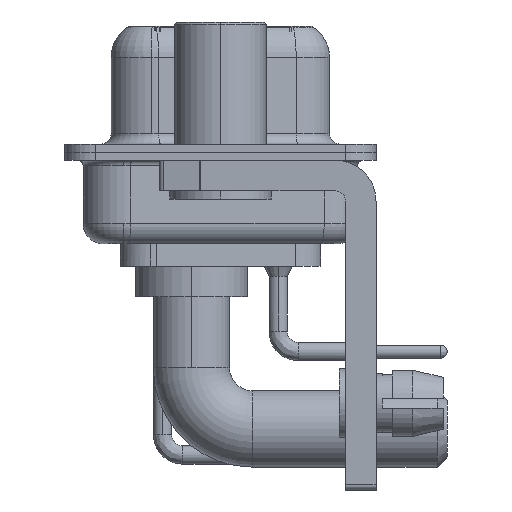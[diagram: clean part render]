
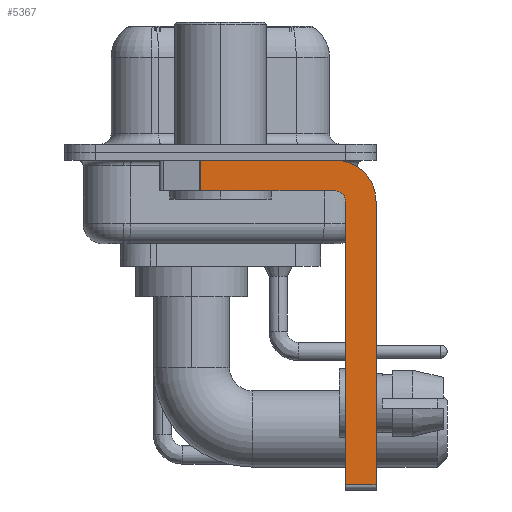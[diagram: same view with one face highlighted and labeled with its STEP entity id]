
A CAD part, left-side view. The second image highlights one B-rep face of the part: STEP entity #5367.
In plain terms, the highlighted planar face has unit normal (-1, 0, 0).
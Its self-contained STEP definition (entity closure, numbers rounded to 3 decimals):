
#263 = ORIENTED_EDGE ( 'NONE', *, *, #15345, .F. ) ;
#335 = EDGE_CURVE ( 'NONE', #21127, #31980, #16540, .T. ) ;
#411 = CARTESIAN_POINT ( 'NONE',  ( -2.9, -5.65, -0.4 ) ) ;
#532 = VERTEX_POINT ( 'NONE', #23320 ) ;
#964 = DIRECTION ( 'NONE',  ( 0., 0., -1. ) ) ;
#1465 = VERTEX_POINT ( 'NONE', #411 ) ;
#1635 = EDGE_CURVE ( 'NONE', #8364, #31980, #29178, .T. ) ;
#1738 = VECTOR ( 'NONE', #964, 1000. ) ;
#2981 = VERTEX_POINT ( 'NONE', #22031 ) ;
#3137 = VERTEX_POINT ( 'NONE', #29108 ) ;
#3294 = EDGE_CURVE ( 'NONE', #30041, #2981, #19776, .T. ) ;
#3747 = DIRECTION ( 'NONE',  ( 1., 0., 0. ) ) ;
#5367 = ADVANCED_FACE ( 'NONE', ( #8749 ), #21542, .F. ) ;
#5401 = ORIENTED_EDGE ( 'NONE', *, *, #16029, .F. ) ;
#5851 = EDGE_CURVE ( 'NONE', #532, #21127, #28391, .T. ) ;
#6353 = DIRECTION ( 'NONE',  ( 0., -1., 0. ) ) ;
#6882 = CIRCLE ( 'NONE', #14861, 2. ) ;
#7047 = LINE ( 'NONE', #24847, #16403 ) ;
#7634 = DIRECTION ( 'NONE',  ( 0., 0., -1. ) ) ;
#8252 = VECTOR ( 'NONE', #19179, 1000. ) ;
#8364 = VERTEX_POINT ( 'NONE', #20105 ) ;
#8749 = FACE_OUTER_BOUND ( 'NONE', #26914, .T. ) ;
#9580 = CARTESIAN_POINT ( 'NONE',  ( -2.9, 0.978, -1.9 ) ) ;
#11492 = DIRECTION ( 'NONE',  ( 0., -1., 0. ) ) ;
#13906 = CARTESIAN_POINT ( 'NONE',  ( -2.9, -5.65, -2.4 ) ) ;
#14336 = LINE ( 'NONE', #31456, #21708 ) ;
#14861 = AXIS2_PLACEMENT_3D ( 'NONE', #30746, #15772, #7634 ) ;
#15345 = EDGE_CURVE ( 'NONE', #8364, #1465, #14336, .T. ) ;
#15772 = DIRECTION ( 'NONE',  ( 1., 0., 0. ) ) ;
#15885 = ORIENTED_EDGE ( 'NONE', *, *, #1635, .T. ) ;
#16029 = EDGE_CURVE ( 'NONE', #1465, #3137, #6882, .T. ) ;
#16403 = VECTOR ( 'NONE', #25015, 1000. ) ;
#16535 = CARTESIAN_POINT ( 'NONE',  ( -2.9, -5.65, -2.4 ) ) ;
#16540 = LINE ( 'NONE', #31331, #8252 ) ;
#16546 = CARTESIAN_POINT ( 'NONE',  ( -2.9, 0.978, -1.9 ) ) ;
#16607 = LINE ( 'NONE', #26745, #1738 ) ;
#16622 = CARTESIAN_POINT ( 'NONE',  ( -2.9, -6.15, -16.35 ) ) ;
#16692 = DIRECTION ( 'NONE',  ( -1., 0., 0. ) ) ;
#17634 = ORIENTED_EDGE ( 'NONE', *, *, #20420, .F. ) ;
#18894 = DIRECTION ( 'NONE',  ( 0., 0., -1. ) ) ;
#19179 = DIRECTION ( 'NONE',  ( 0., 1., 0. ) ) ;
#19776 = LINE ( 'NONE', #26616, #20875 ) ;
#20105 = CARTESIAN_POINT ( 'NONE',  ( -2.9, 0.978, -0.4 ) ) ;
#20420 = EDGE_CURVE ( 'NONE', #3137, #2981, #16607, .T. ) ;
#20875 = VECTOR ( 'NONE', #11492, 1000. ) ;
#21127 = VERTEX_POINT ( 'NONE', #30826 ) ;
#21197 = ORIENTED_EDGE ( 'NONE', *, *, #30453, .F. ) ;
#21542 = PLANE ( 'NONE',  #28367 ) ;
#21708 = VECTOR ( 'NONE', #6353, 1000. ) ;
#22031 = CARTESIAN_POINT ( 'NONE',  ( -2.9, -7.65, -16.35 ) ) ;
#22706 = ORIENTED_EDGE ( 'NONE', *, *, #335, .F. ) ;
#23320 = CARTESIAN_POINT ( 'NONE',  ( -2.9, -6.15, -2.4 ) ) ;
#24133 = AXIS2_PLACEMENT_3D ( 'NONE', #16535, #16692, #26990 ) ;
#24786 = VECTOR ( 'NONE', #26671, 1000. ) ;
#24847 = CARTESIAN_POINT ( 'NONE',  ( -2.9, -6.15, -16.6 ) ) ;
#25015 = DIRECTION ( 'NONE',  ( 0., 0., 1. ) ) ;
#26616 = CARTESIAN_POINT ( 'NONE',  ( -2.9, -5.65, -16.35 ) ) ;
#26671 = DIRECTION ( 'NONE',  ( 0., 0., -1. ) ) ;
#26745 = CARTESIAN_POINT ( 'NONE',  ( -2.9, -7.65, -2.4 ) ) ;
#26914 = EDGE_LOOP ( 'NONE', ( #263, #15885, #22706, #32028, #21197, #28468, #17634, #5401 ) ) ;
#26990 = DIRECTION ( 'NONE',  ( 0., 0., 1. ) ) ;
#28367 = AXIS2_PLACEMENT_3D ( 'NONE', #13906, #3747, #18894 ) ;
#28391 = CIRCLE ( 'NONE', #24133, 0.5 ) ;
#28468 = ORIENTED_EDGE ( 'NONE', *, *, #3294, .T. ) ;
#29108 = CARTESIAN_POINT ( 'NONE',  ( -2.9, -7.65, -2.4 ) ) ;
#29178 = LINE ( 'NONE', #16546, #24786 ) ;
#30041 = VERTEX_POINT ( 'NONE', #16622 ) ;
#30453 = EDGE_CURVE ( 'NONE', #30041, #532, #7047, .T. ) ;
#30746 = CARTESIAN_POINT ( 'NONE',  ( -2.9, -5.65, -2.4 ) ) ;
#30826 = CARTESIAN_POINT ( 'NONE',  ( -2.9, -5.65, -1.9 ) ) ;
#31331 = CARTESIAN_POINT ( 'NONE',  ( -2.9, -5.65, -1.9 ) ) ;
#31456 = CARTESIAN_POINT ( 'NONE',  ( -2.9, 3., -0.4 ) ) ;
#31980 = VERTEX_POINT ( 'NONE', #9580 ) ;
#32028 = ORIENTED_EDGE ( 'NONE', *, *, #5851, .F. ) ;
